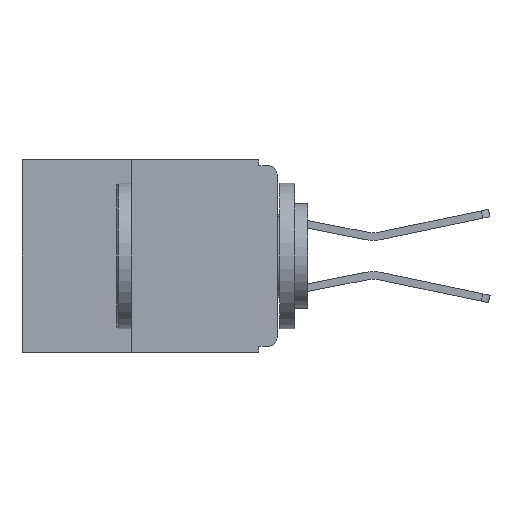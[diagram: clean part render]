
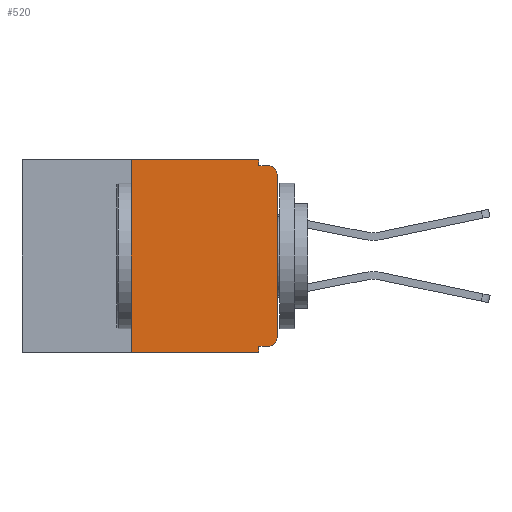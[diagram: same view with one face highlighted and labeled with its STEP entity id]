
A CAD part, left-side view. The second image highlights one B-rep face of the part: STEP entity #520.
In plain terms, the highlighted planar face has unit normal (-1, 0, 0).
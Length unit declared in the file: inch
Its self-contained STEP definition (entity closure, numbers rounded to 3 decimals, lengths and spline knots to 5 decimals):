
#358 = VERTEX_POINT ( 'NONE', #1154 ) ;
#520 = ADVANCED_FACE ( 'NONE', ( #3501 ), #9954, .F. ) ;
#561 = CARTESIAN_POINT ( 'NONE',  ( 0., 0.437, -0.33 ) ) ;
#709 = ORIENTED_EDGE ( 'NONE', *, *, #1097, .T. ) ;
#833 = ORIENTED_EDGE ( 'NONE', *, *, #14975, .T. ) ;
#1047 = CARTESIAN_POINT ( 'NONE',  ( 0., 0.25, 0. ) ) ;
#1097 = EDGE_CURVE ( 'NONE', #15678, #6674, #10273, .T. ) ;
#1154 = CARTESIAN_POINT ( 'NONE',  ( 0., 0.031, -0.32 ) ) ;
#1361 = VERTEX_POINT ( 'NONE', #4353 ) ;
#1570 = VERTEX_POINT ( 'NONE', #15555 ) ;
#1634 = ORIENTED_EDGE ( 'NONE', *, *, #12458, .F. ) ;
#1736 = VERTEX_POINT ( 'NONE', #12541 ) ;
#1782 = ORIENTED_EDGE ( 'NONE', *, *, #7060, .F. ) ;
#1813 = ORIENTED_EDGE ( 'NONE', *, *, #19452, .F. ) ;
#2070 = ORIENTED_EDGE ( 'NONE', *, *, #7985, .F. ) ;
#2089 = ORIENTED_EDGE ( 'NONE', *, *, #16869, .T. ) ;
#2192 = DIRECTION ( 'NONE',  ( 0., 0., 1. ) ) ;
#2214 = DIRECTION ( 'NONE',  ( 0., -1., 0. ) ) ;
#2231 = VECTOR ( 'NONE', #2214, 39.37008 ) ;
#2335 = CARTESIAN_POINT ( 'NONE',  ( 0., 0., -0.01 ) ) ;
#2340 = ORIENTED_EDGE ( 'NONE', *, *, #18730, .F. ) ;
#2426 = DIRECTION ( 'NONE',  ( 0., 0., 1. ) ) ;
#2479 = CARTESIAN_POINT ( 'NONE',  ( 0., 0.25, -0.33 ) ) ;
#2532 = DIRECTION ( 'NONE',  ( 0., 0., -1. ) ) ;
#2945 = DIRECTION ( 'NONE',  ( -1., 0., 0. ) ) ;
#2992 = CARTESIAN_POINT ( 'NONE',  ( 0., 0.015, -0.305 ) ) ;
#3315 = CIRCLE ( 'NONE', #5153, 0.015 ) ;
#3324 = ORIENTED_EDGE ( 'NONE', *, *, #5863, .F. ) ;
#3370 = DIRECTION ( 'NONE',  ( 0., -1., 0. ) ) ;
#3501 = FACE_OUTER_BOUND ( 'NONE', #5470, .T. ) ;
#3526 = DIRECTION ( 'NONE',  ( 0., 0., -1. ) ) ;
#4161 = LINE ( 'NONE', #15690, #19669 ) ;
#4353 = CARTESIAN_POINT ( 'NONE',  ( 0., 0.015, -0.01 ) ) ;
#5153 = AXIS2_PLACEMENT_3D ( 'NONE', #17947, #9073, #19433 ) ;
#5385 = CARTESIAN_POINT ( 'NONE',  ( 0., 0.437, 0. ) ) ;
#5470 = EDGE_LOOP ( 'NONE', ( #709, #833, #1634, #1782, #1813, #2070, #2089, #2340, #3324, #9488 ) ) ;
#5831 = DIRECTION ( 'NONE',  ( 1., 0., 0. ) ) ;
#5863 = EDGE_CURVE ( 'NONE', #10287, #358, #8091, .T. ) ;
#6604 = AXIS2_PLACEMENT_3D ( 'NONE', #5385, #5831, #3526 ) ;
#6674 = VERTEX_POINT ( 'NONE', #15877 ) ;
#6827 = VECTOR ( 'NONE', #12035, 39.37008 ) ;
#7060 = EDGE_CURVE ( 'NONE', #1570, #1736, #14815, .T. ) ;
#7075 = CIRCLE ( 'NONE', #8369, 0.015 ) ;
#7573 = LINE ( 'NONE', #2335, #14607 ) ;
#7756 = CARTESIAN_POINT ( 'NONE',  ( 0., 0.015, -0.32 ) ) ;
#7985 = EDGE_CURVE ( 'NONE', #8411, #15482, #11337, .T. ) ;
#8091 = LINE ( 'NONE', #11175, #15533 ) ;
#8293 = DIRECTION ( 'NONE',  ( 0., 0., -1. ) ) ;
#8359 = CARTESIAN_POINT ( 'NONE',  ( 0., 0.031, -0.33 ) ) ;
#8369 = AXIS2_PLACEMENT_3D ( 'NONE', #2992, #2945, #2532 ) ;
#8411 = VERTEX_POINT ( 'NONE', #15991 ) ;
#9073 = DIRECTION ( 'NONE',  ( -1., 0., 0. ) ) ;
#9395 = CARTESIAN_POINT ( 'NONE',  ( 0., 0., -0.305 ) ) ;
#9488 = ORIENTED_EDGE ( 'NONE', *, *, #12437, .T. ) ;
#9573 = DIRECTION ( 'NONE',  ( 0., -1., 0. ) ) ;
#9954 = PLANE ( 'NONE',  #6604 ) ;
#10273 = LINE ( 'NONE', #12611, #10736 ) ;
#10287 = VERTEX_POINT ( 'NONE', #7756 ) ;
#10640 = LINE ( 'NONE', #16940, #18015 ) ;
#10736 = VECTOR ( 'NONE', #2426, 39.37008 ) ;
#11175 = CARTESIAN_POINT ( 'NONE',  ( 0., 0., -0.32 ) ) ;
#11253 = DIRECTION ( 'NONE',  ( 0., 1., 0. ) ) ;
#11337 = LINE ( 'NONE', #2479, #14320 ) ;
#11579 = CARTESIAN_POINT ( 'NONE',  ( 0., 0.031, 0. ) ) ;
#12035 = DIRECTION ( 'NONE',  ( 0., 0., -1. ) ) ;
#12437 = EDGE_CURVE ( 'NONE', #10287, #15678, #7075, .T. ) ;
#12458 = EDGE_CURVE ( 'NONE', #1736, #1361, #7573, .T. ) ;
#12541 = CARTESIAN_POINT ( 'NONE',  ( 0., 0.031, -0.01 ) ) ;
#12611 = CARTESIAN_POINT ( 'NONE',  ( 0., 0., 0. ) ) ;
#14320 = VECTOR ( 'NONE', #2192, 39.37008 ) ;
#14401 = LINE ( 'NONE', #561, #2231 ) ;
#14607 = VECTOR ( 'NONE', #3370, 39.37008 ) ;
#14711 = VERTEX_POINT ( 'NONE', #8359 ) ;
#14815 = LINE ( 'NONE', #11579, #6827 ) ;
#14975 = EDGE_CURVE ( 'NONE', #6674, #1361, #3315, .T. ) ;
#15482 = VERTEX_POINT ( 'NONE', #1047 ) ;
#15533 = VECTOR ( 'NONE', #11253, 39.37008 ) ;
#15555 = CARTESIAN_POINT ( 'NONE',  ( 0., 0.031, 0. ) ) ;
#15678 = VERTEX_POINT ( 'NONE', #9395 ) ;
#15690 = CARTESIAN_POINT ( 'NONE',  ( 0., 0.031, -0.33 ) ) ;
#15877 = CARTESIAN_POINT ( 'NONE',  ( 0., 0., -0.025 ) ) ;
#15991 = CARTESIAN_POINT ( 'NONE',  ( 0., 0.25, -0.33 ) ) ;
#16869 = EDGE_CURVE ( 'NONE', #8411, #14711, #14401, .T. ) ;
#16940 = CARTESIAN_POINT ( 'NONE',  ( 0., 0.437, 0. ) ) ;
#17947 = CARTESIAN_POINT ( 'NONE',  ( 0., 0.015, -0.025 ) ) ;
#18015 = VECTOR ( 'NONE', #9573, 39.37008 ) ;
#18730 = EDGE_CURVE ( 'NONE', #358, #14711, #4161, .T. ) ;
#19433 = DIRECTION ( 'NONE',  ( 0., 0., -1. ) ) ;
#19452 = EDGE_CURVE ( 'NONE', #15482, #1570, #10640, .T. ) ;
#19669 = VECTOR ( 'NONE', #8293, 39.37008 ) ;
